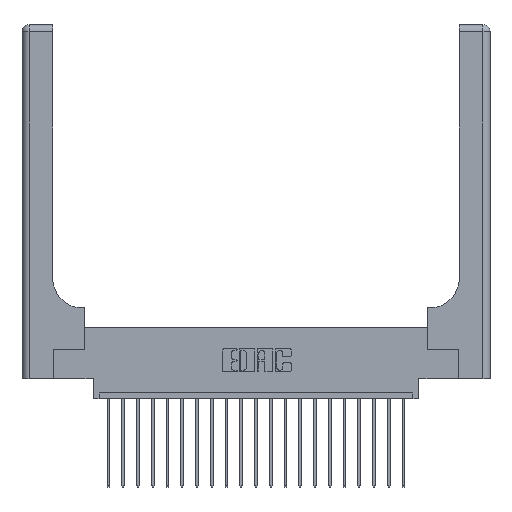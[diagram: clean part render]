
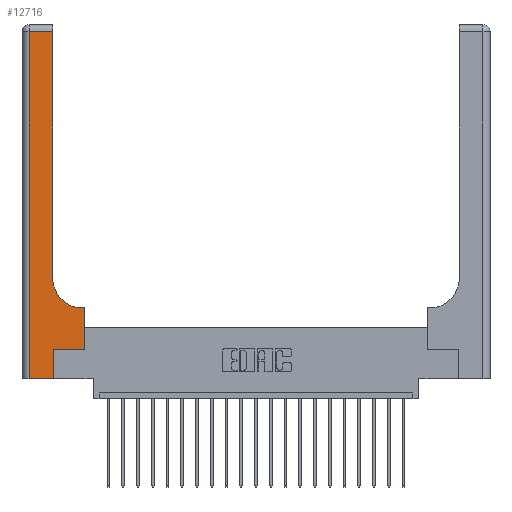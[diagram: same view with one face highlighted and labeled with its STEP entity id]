
A CAD part, top view. The second image highlights one B-rep face of the part: STEP entity #12716.
In plain terms, the highlighted planar face has unit normal (0, 0, 1).
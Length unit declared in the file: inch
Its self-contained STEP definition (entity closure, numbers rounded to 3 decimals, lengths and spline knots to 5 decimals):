
#47 = DIRECTION ( 'NONE',  ( 1., 0., 0. ) ) ;
#262 = DIRECTION ( 'NONE',  ( 1., 0., 0. ) ) ;
#418 = CARTESIAN_POINT ( 'NONE',  ( 0.265, 0.25, 0.37 ) ) ;
#811 = VECTOR ( 'NONE', #11918, 39.37008 ) ;
#949 = VERTEX_POINT ( 'NONE', #10720 ) ;
#1044 = ORIENTED_EDGE ( 'NONE', *, *, #19056, .T. ) ;
#1118 = VERTEX_POINT ( 'NONE', #418 ) ;
#1307 = CARTESIAN_POINT ( 'NONE',  ( 0.06, 3., 0.37 ) ) ;
#2488 = LINE ( 'NONE', #4064, #12231 ) ;
#3551 = ORIENTED_EDGE ( 'NONE', *, *, #20520, .T. ) ;
#3739 = EDGE_CURVE ( 'NONE', #9982, #20461, #19933, .T. ) ;
#3994 = VECTOR ( 'NONE', #262, 39.37008 ) ;
#4023 = DIRECTION ( 'NONE',  ( -1., 0., 0. ) ) ;
#4064 = CARTESIAN_POINT ( 'NONE',  ( 0.265, 0., 0.37 ) ) ;
#4174 = ORIENTED_EDGE ( 'NONE', *, *, #5619, .T. ) ;
#4224 = VECTOR ( 'NONE', #19985, 39.37008 ) ;
#4647 = CARTESIAN_POINT ( 'NONE',  ( 0.06, 2.94, 0.37 ) ) ;
#4806 = AXIS2_PLACEMENT_3D ( 'NONE', #13352, #20021, #47 ) ;
#5584 = CARTESIAN_POINT ( 'NONE',  ( 0.51, 0.6, 0.37 ) ) ;
#5619 = EDGE_CURVE ( 'NONE', #949, #20921, #10837, .T. ) ;
#5727 = VERTEX_POINT ( 'NONE', #20086 ) ;
#5813 = PLANE ( 'NONE',  #13902 ) ;
#6697 = EDGE_CURVE ( 'NONE', #20921, #14837, #15421, .T. ) ;
#6954 = EDGE_CURVE ( 'NONE', #20461, #5727, #16169, .T. ) ;
#7023 = CARTESIAN_POINT ( 'NONE',  ( 0.26, 0.85, 0.37 ) ) ;
#7333 = DIRECTION ( 'NONE',  ( 0., 0., -1. ) ) ;
#7925 = DIRECTION ( 'NONE',  ( 0., -1., 0. ) ) ;
#8722 = CARTESIAN_POINT ( 'NONE',  ( 0.265, 0., 0.37 ) ) ;
#9385 = LINE ( 'NONE', #18425, #3994 ) ;
#9982 = VERTEX_POINT ( 'NONE', #16598 ) ;
#10418 = FACE_OUTER_BOUND ( 'NONE', #20103, .T. ) ;
#10446 = CARTESIAN_POINT ( 'NONE',  ( 0.26, 3., 0.37 ) ) ;
#10611 = ORIENTED_EDGE ( 'NONE', *, *, #13065, .T. ) ;
#10720 = CARTESIAN_POINT ( 'NONE',  ( 0.528, 0.25, 0.37 ) ) ;
#10837 = LINE ( 'NONE', #15139, #11091 ) ;
#10878 = CARTESIAN_POINT ( 'NONE',  ( 0.528, 0.6, 0.37 ) ) ;
#11091 = VECTOR ( 'NONE', #15206, 39.37008 ) ;
#11379 = EDGE_CURVE ( 'NONE', #1118, #949, #18955, .T. ) ;
#11918 = DIRECTION ( 'NONE',  ( -1., 0., 0. ) ) ;
#12024 = CARTESIAN_POINT ( 'NONE',  ( 0.265, 0.25, 0.37 ) ) ;
#12123 = DIRECTION ( 'NONE',  ( 0., 1., 0. ) ) ;
#12231 = VECTOR ( 'NONE', #12123, 39.37008 ) ;
#12370 = ORIENTED_EDGE ( 'NONE', *, *, #6954, .T. ) ;
#12428 = CARTESIAN_POINT ( 'NONE',  ( 0., 3., 0.37 ) ) ;
#12716 = ADVANCED_FACE ( 'NONE', ( #10418 ), #5813, .F. ) ;
#13065 = EDGE_CURVE ( 'NONE', #5727, #21190, #9385, .T. ) ;
#13090 = CARTESIAN_POINT ( 'NONE',  ( 0.26, 0.6, 0.37 ) ) ;
#13352 = CARTESIAN_POINT ( 'NONE',  ( 0.51, 0.85, 0.37 ) ) ;
#13902 = AXIS2_PLACEMENT_3D ( 'NONE', #12428, #7333, #4023 ) ;
#13965 = DIRECTION ( 'NONE',  ( 0., 1., 0. ) ) ;
#14242 = DIRECTION ( 'NONE',  ( 1., 0., 0. ) ) ;
#14276 = LINE ( 'NONE', #10446, #19391 ) ;
#14837 = VERTEX_POINT ( 'NONE', #5584 ) ;
#15139 = CARTESIAN_POINT ( 'NONE',  ( 0.528, 0.25, 0.37 ) ) ;
#15206 = DIRECTION ( 'NONE',  ( 0., 1., 0. ) ) ;
#15421 = LINE ( 'NONE', #13090, #811 ) ;
#16169 = LINE ( 'NONE', #1307, #20543 ) ;
#16598 = CARTESIAN_POINT ( 'NONE',  ( 0.26, 2.94, 0.37 ) ) ;
#18266 = ORIENTED_EDGE ( 'NONE', *, *, #19378, .T. ) ;
#18425 = CARTESIAN_POINT ( 'NONE',  ( 0., 0., 0.37 ) ) ;
#18440 = ORIENTED_EDGE ( 'NONE', *, *, #6697, .T. ) ;
#18592 = CARTESIAN_POINT ( 'NONE',  ( 0., 2.94, 0.37 ) ) ;
#18955 = LINE ( 'NONE', #12024, #20256 ) ;
#19003 = VERTEX_POINT ( 'NONE', #7023 ) ;
#19056 = EDGE_CURVE ( 'NONE', #21190, #1118, #2488, .T. ) ;
#19079 = CIRCLE ( 'NONE', #4806, 0.25 ) ;
#19378 = EDGE_CURVE ( 'NONE', #19003, #9982, #14276, .T. ) ;
#19391 = VECTOR ( 'NONE', #13965, 39.37008 ) ;
#19817 = ORIENTED_EDGE ( 'NONE', *, *, #11379, .T. ) ;
#19823 = ORIENTED_EDGE ( 'NONE', *, *, #3739, .T. ) ;
#19933 = LINE ( 'NONE', #18592, #4224 ) ;
#19985 = DIRECTION ( 'NONE',  ( -1., 0., 0. ) ) ;
#20021 = DIRECTION ( 'NONE',  ( 0., 0., -1. ) ) ;
#20086 = CARTESIAN_POINT ( 'NONE',  ( 0.06, 0., 0.37 ) ) ;
#20103 = EDGE_LOOP ( 'NONE', ( #18266, #19823, #12370, #10611, #1044, #19817, #4174, #18440, #3551 ) ) ;
#20256 = VECTOR ( 'NONE', #14242, 39.37008 ) ;
#20461 = VERTEX_POINT ( 'NONE', #4647 ) ;
#20520 = EDGE_CURVE ( 'NONE', #14837, #19003, #19079, .T. ) ;
#20543 = VECTOR ( 'NONE', #7925, 39.37008 ) ;
#20921 = VERTEX_POINT ( 'NONE', #10878 ) ;
#21190 = VERTEX_POINT ( 'NONE', #8722 ) ;
